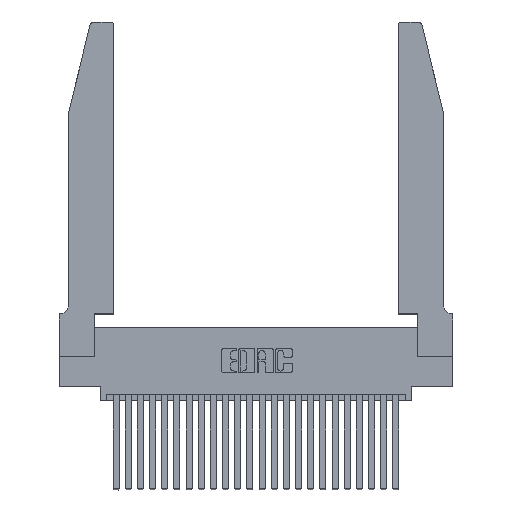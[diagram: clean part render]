
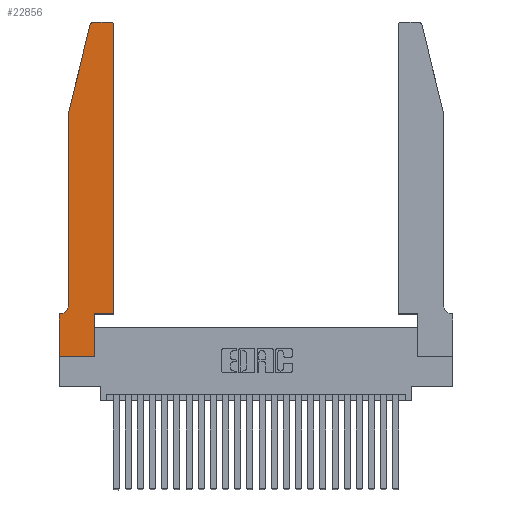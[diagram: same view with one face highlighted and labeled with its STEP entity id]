
A CAD part, top view. The second image highlights one B-rep face of the part: STEP entity #22856.
In plain terms, the highlighted planar face has unit normal (0, 0, 1).
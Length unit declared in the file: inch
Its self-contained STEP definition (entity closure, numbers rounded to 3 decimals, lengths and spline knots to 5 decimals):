
#11 = VERTEX_POINT ( 'NONE', #434 ) ;
#106 = VERTEX_POINT ( 'NONE', #22896 ) ;
#335 = CARTESIAN_POINT ( 'NONE',  ( 0., 0.35, 0.37 ) ) ;
#434 = CARTESIAN_POINT ( 'NONE',  ( 0., 0., 0.37 ) ) ;
#709 = DIRECTION ( 'NONE',  ( 0., 1., 0. ) ) ;
#1172 = DIRECTION ( 'NONE',  ( -0.239, -0.971, 0. ) ) ;
#2276 = VERTEX_POINT ( 'NONE', #20052 ) ;
#2317 = VECTOR ( 'NONE', #23688, 39.37008 ) ;
#2463 = VERTEX_POINT ( 'NONE', #21250 ) ;
#2632 = LINE ( 'NONE', #13548, #2317 ) ;
#2647 = CARTESIAN_POINT ( 'NONE',  ( 0.4505, 0.35, 0.37 ) ) ;
#2663 = ORIENTED_EDGE ( 'NONE', *, *, #24431, .T. ) ;
#2692 = CARTESIAN_POINT ( 'NONE',  ( 0., 0., 0.37 ) ) ;
#2735 = DIRECTION ( 'NONE',  ( 0., -1., 0. ) ) ;
#3130 = CARTESIAN_POINT ( 'NONE',  ( 0.4205, 2.72, 0.37 ) ) ;
#3697 = VECTOR ( 'NONE', #2735, 39.37008 ) ;
#3725 = VERTEX_POINT ( 'NONE', #9153 ) ;
#4694 = VERTEX_POINT ( 'NONE', #15500 ) ;
#5015 = LINE ( 'NONE', #17098, #7851 ) ;
#5036 = VERTEX_POINT ( 'NONE', #17002 ) ;
#5280 = CARTESIAN_POINT ( 'NONE',  ( 0.4505, 0.35, 0.37 ) ) ;
#5466 = CARTESIAN_POINT ( 'NONE',  ( 0.284, 2.75, 0.37 ) ) ;
#5717 = CARTESIAN_POINT ( 'NONE',  ( 0., 0.35, 0.37 ) ) ;
#5913 = DIRECTION ( 'NONE',  ( 0., 0., -1. ) ) ;
#6516 = EDGE_CURVE ( 'NONE', #11, #2463, #11485, .T. ) ;
#6621 = ORIENTED_EDGE ( 'NONE', *, *, #25556, .T. ) ;
#7008 = VERTEX_POINT ( 'NONE', #16338 ) ;
#7851 = VECTOR ( 'NONE', #1172, 39.37008 ) ;
#8320 = ORIENTED_EDGE ( 'NONE', *, *, #6516, .T. ) ;
#8364 = PLANE ( 'NONE',  #17715 ) ;
#8655 = ORIENTED_EDGE ( 'NONE', *, *, #25643, .T. ) ;
#8999 = ORIENTED_EDGE ( 'NONE', *, *, #21881, .T. ) ;
#9133 = CARTESIAN_POINT ( 'NONE',  ( 0.284, 2.72, 0.37 ) ) ;
#9149 = LINE ( 'NONE', #5280, #22609 ) ;
#9153 = CARTESIAN_POINT ( 'NONE',  ( 0.4205, 2.75, 0.37 ) ) ;
#9341 = EDGE_CURVE ( 'NONE', #3725, #21322, #25742, .T. ) ;
#9745 = ORIENTED_EDGE ( 'NONE', *, *, #9341, .T. ) ;
#10015 = EDGE_LOOP ( 'NONE', ( #9745, #2663, #24400, #6621, #13281, #8655, #13728, #8320, #17024, #22617, #21902, #8999 ) ) ;
#10125 = EDGE_CURVE ( 'NONE', #11595, #4694, #5015, .T. ) ;
#10187 = CIRCLE ( 'NONE', #24050, 0.07 ) ;
#10477 = CARTESIAN_POINT ( 'NONE',  ( 0., 0., 0.37 ) ) ;
#11191 = VERTEX_POINT ( 'NONE', #5717 ) ;
#11430 = DIRECTION ( 'NONE',  ( -1., 0., 0. ) ) ;
#11485 = LINE ( 'NONE', #10477, #21548 ) ;
#11558 = LINE ( 'NONE', #2647, #18807 ) ;
#11595 = VERTEX_POINT ( 'NONE', #16629 ) ;
#11963 = AXIS2_PLACEMENT_3D ( 'NONE', #9133, #23153, #18887 ) ;
#12709 = VERTEX_POINT ( 'NONE', #24040 ) ;
#12795 = DIRECTION ( 'NONE',  ( 1., 0., 0. ) ) ;
#13250 = EDGE_CURVE ( 'NONE', #2463, #106, #2632, .T. ) ;
#13281 = ORIENTED_EDGE ( 'NONE', *, *, #16992, .T. ) ;
#13548 = CARTESIAN_POINT ( 'NONE',  ( 0.2865, 0.35, 0.37 ) ) ;
#13728 = ORIENTED_EDGE ( 'NONE', *, *, #21777, .T. ) ;
#14609 = DIRECTION ( 'NONE',  ( 1., 0., 0. ) ) ;
#14736 = VECTOR ( 'NONE', #11430, 39.37008 ) ;
#15193 = AXIS2_PLACEMENT_3D ( 'NONE', #3130, #25396, #25143 ) ;
#15425 = CIRCLE ( 'NONE', #11963, 0.03 ) ;
#15453 = VECTOR ( 'NONE', #18088, 39.37008 ) ;
#15500 = CARTESIAN_POINT ( 'NONE',  ( 0.0755, 2., 0.37 ) ) ;
#15911 = FACE_OUTER_BOUND ( 'NONE', #10015, .T. ) ;
#16071 = CARTESIAN_POINT ( 'NONE',  ( 0.2605, 2.75, 0.37 ) ) ;
#16269 = LINE ( 'NONE', #19009, #3697 ) ;
#16338 = CARTESIAN_POINT ( 'NONE',  ( 0.0055, 0.35, 0.37 ) ) ;
#16583 = LINE ( 'NONE', #2692, #24391 ) ;
#16629 = CARTESIAN_POINT ( 'NONE',  ( 0.25487, 2.72718, 0.37 ) ) ;
#16992 = EDGE_CURVE ( 'NONE', #12709, #7008, #10187, .T. ) ;
#17002 = CARTESIAN_POINT ( 'NONE',  ( 0.4505, 0.35, 0.37 ) ) ;
#17024 = ORIENTED_EDGE ( 'NONE', *, *, #13250, .T. ) ;
#17098 = CARTESIAN_POINT ( 'NONE',  ( 0.0755, 2., 0.37 ) ) ;
#17715 = AXIS2_PLACEMENT_3D ( 'NONE', #335, #20477, #14609 ) ;
#17949 = CARTESIAN_POINT ( 'NONE',  ( 0.0055, 0.42, 0.37 ) ) ;
#18088 = DIRECTION ( 'NONE',  ( -1., 0., 0. ) ) ;
#18807 = VECTOR ( 'NONE', #709, 39.37008 ) ;
#18887 = DIRECTION ( 'NONE',  ( 1., 0., 0. ) ) ;
#19009 = CARTESIAN_POINT ( 'NONE',  ( 0.0755, 2., 0.37 ) ) ;
#19395 = EDGE_CURVE ( 'NONE', #106, #5036, #9149, .T. ) ;
#20052 = CARTESIAN_POINT ( 'NONE',  ( 0.4505, 2.72, 0.37 ) ) ;
#20477 = DIRECTION ( 'NONE',  ( 0., 0., 1. ) ) ;
#21033 = CARTESIAN_POINT ( 'NONE',  ( 0.0755, 0.35, 0.37 ) ) ;
#21250 = CARTESIAN_POINT ( 'NONE',  ( 0.2865, 0., 0.37 ) ) ;
#21322 = VERTEX_POINT ( 'NONE', #5466 ) ;
#21548 = VECTOR ( 'NONE', #12795, 39.37008 ) ;
#21777 = EDGE_CURVE ( 'NONE', #11191, #11, #16583, .T. ) ;
#21881 = EDGE_CURVE ( 'NONE', #2276, #3725, #25947, .T. ) ;
#21902 = ORIENTED_EDGE ( 'NONE', *, *, #25605, .T. ) ;
#22185 = DIRECTION ( 'NONE',  ( -1., 0., 0. ) ) ;
#22205 = LINE ( 'NONE', #21033, #14736 ) ;
#22609 = VECTOR ( 'NONE', #23428, 39.37008 ) ;
#22617 = ORIENTED_EDGE ( 'NONE', *, *, #19395, .T. ) ;
#22776 = DIRECTION ( 'NONE',  ( 0., -1., 0. ) ) ;
#22856 = ADVANCED_FACE ( 'NONE', ( #15911 ), #8364, .T. ) ;
#22896 = CARTESIAN_POINT ( 'NONE',  ( 0.2865, 0.35, 0.37 ) ) ;
#23153 = DIRECTION ( 'NONE',  ( 0., 0., 1. ) ) ;
#23428 = DIRECTION ( 'NONE',  ( 1., 0., 0. ) ) ;
#23688 = DIRECTION ( 'NONE',  ( 0., 1., 0. ) ) ;
#24040 = CARTESIAN_POINT ( 'NONE',  ( 0.0755, 0.42, 0.37 ) ) ;
#24050 = AXIS2_PLACEMENT_3D ( 'NONE', #17949, #5913, #22185 ) ;
#24391 = VECTOR ( 'NONE', #22776, 39.37008 ) ;
#24400 = ORIENTED_EDGE ( 'NONE', *, *, #10125, .T. ) ;
#24431 = EDGE_CURVE ( 'NONE', #21322, #11595, #15425, .T. ) ;
#25143 = DIRECTION ( 'NONE',  ( 1., 0., 0. ) ) ;
#25396 = DIRECTION ( 'NONE',  ( 0., 0., 1. ) ) ;
#25556 = EDGE_CURVE ( 'NONE', #4694, #12709, #16269, .T. ) ;
#25605 = EDGE_CURVE ( 'NONE', #5036, #2276, #11558, .T. ) ;
#25643 = EDGE_CURVE ( 'NONE', #7008, #11191, #22205, .T. ) ;
#25742 = LINE ( 'NONE', #16071, #15453 ) ;
#25947 = CIRCLE ( 'NONE', #15193, 0.03 ) ;
